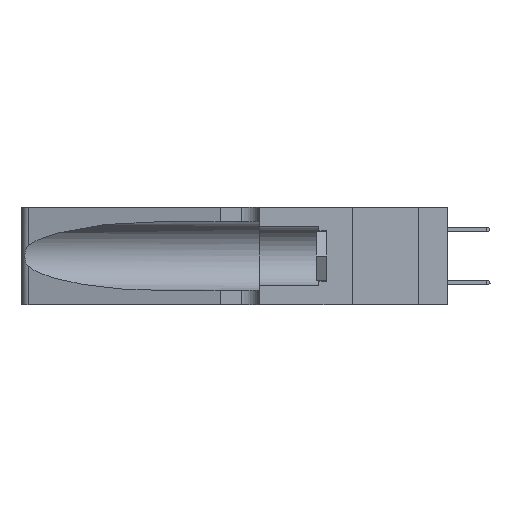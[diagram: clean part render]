
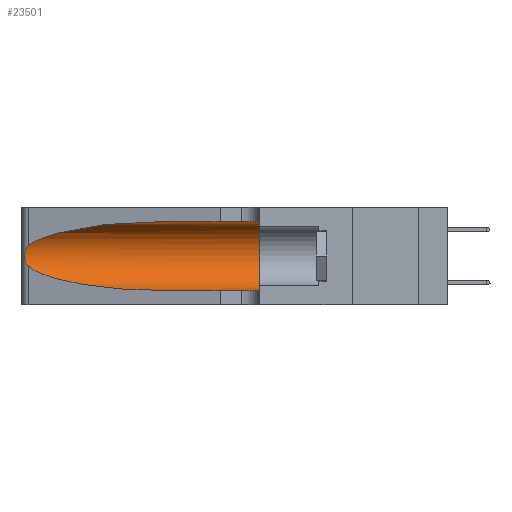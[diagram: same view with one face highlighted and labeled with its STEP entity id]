
A CAD part, left-side view. The second image highlights one B-rep face of the part: STEP entity #23501.
In plain terms, the highlighted cylindrical face has radius 3.308 mm (diameter 6.617 mm), a partial arc.
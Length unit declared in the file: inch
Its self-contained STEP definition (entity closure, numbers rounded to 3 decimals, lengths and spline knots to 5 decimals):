
#346 = CARTESIAN_POINT ( 'NONE',  ( 0.18966, 0.96281, 0.05475 ) ) ;
#382 = CARTESIAN_POINT ( 'NONE',  ( 0.1305, 1.61858, 0.185 ) ) ;
#790 = CARTESIAN_POINT ( 'NONE',  ( 0.1305, 0.72297, 0.31525 ) ) ;
#929 = CARTESIAN_POINT ( 'NONE',  ( 0.25789, 1.23486, 0.15765 ) ) ;
#1046 = CARTESIAN_POINT ( 'NONE',  ( 0.26075, 1.23896, 0.19203 ) ) ;
#2402 = ORIENTED_EDGE ( 'NONE', *, *, #20132, .F. ) ;
#3681 = VECTOR ( 'NONE', #14941, 39.37008 ) ;
#4393 = CARTESIAN_POINT ( 'NONE',  ( 0.25487, 1.22718, 0.22369 ) ) ;
#5688 = CARTESIAN_POINT ( 'NONE',  ( 0.1305, 0.72297, 0.05475 ) ) ;
#6216 = CARTESIAN_POINT ( 'NONE',  ( 0.1305, 1.61858, 0.31525 ) ) ;
#6622 = CARTESIAN_POINT ( 'NONE',  ( 0.25639, 1.23186, 0.15144 ) ) ;
#6860 = CARTESIAN_POINT ( 'NONE',  ( 0.1305, 0.35, 0.185 ) ) ;
#9058 = ORIENTED_EDGE ( 'NONE', *, *, #12781, .T. ) ;
#9461 = CARTESIAN_POINT ( 'NONE',  ( 0.25639, 1.23184, 0.21858 ) ) ;
#9707 = DIRECTION ( 'NONE',  ( 0., 1., 0. ) ) ;
#9995 = ORIENTED_EDGE ( 'NONE', *, *, #31257, .F. ) ;
#11480 = CARTESIAN_POINT ( 'NONE',  ( 0.2373, 1.15595, 0.08982 ) ) ;
#11540 = CARTESIAN_POINT ( 'NONE',  ( 0.1305, 0.72297, 0.31525 ) ) ;
#11659 = CARTESIAN_POINT ( 'NONE',  ( 0.1305, 0.35, 0.05475 ) ) ;
#12025 = CARTESIAN_POINT ( 'NONE',  ( 0.25555, 1.22993, 0.14849 ) ) ;
#12149 = CARTESIAN_POINT ( 'NONE',  ( 0.25854, 1.2359, 0.20912 ) ) ;
#12541 = LINE ( 'NONE', #15565, #25305 ) ;
#12622 = EDGE_CURVE ( 'NONE', #35712, #19726, #35573, .T. ) ;
#12781 = EDGE_CURVE ( 'NONE', #19726, #19125, #35124, .T. ) ;
#12976 = AXIS2_PLACEMENT_3D ( 'NONE', #6860, #9707, #29433 ) ;
#13161 = CARTESIAN_POINT ( 'NONE',  ( 0.1305, 0.35, 0.31525 ) ) ;
#14578 = VERTEX_POINT ( 'NONE', #11659 ) ;
#14941 = DIRECTION ( 'NONE',  ( 0., -1., 0. ) ) ;
#15565 = CARTESIAN_POINT ( 'NONE',  ( 0.1305, 1.61858, 0.05475 ) ) ;
#16082 = EDGE_CURVE ( 'NONE', #19125, #25870, #28475, .T. ) ;
#16121 = EDGE_LOOP ( 'NONE', ( #23765, #9058, #29071, #16289, #9995, #2402 ) ) ;
#16289 = ORIENTED_EDGE ( 'NONE', *, *, #34097, .T. ) ;
#16710 = CARTESIAN_POINT ( 'NONE',  ( 0.1305, 0.72297, 0.05475 ) ) ;
#17772 = DIRECTION ( 'NONE',  ( 0., -1., 0. ) ) ;
#18068 = CARTESIAN_POINT ( 'NONE',  ( 0.25787, 1.23484, 0.2124 ) ) ;
#19125 = VERTEX_POINT ( 'NONE', #36309 ) ;
#19726 = VERTEX_POINT ( 'NONE', #4393 ) ;
#20132 = EDGE_CURVE ( 'NONE', #35712, #32772, #32835, .T. ) ;
#23467 = CARTESIAN_POINT ( 'NONE',  ( 0.25555, 1.22994, 0.2215 ) ) ;
#23501 = ADVANCED_FACE ( 'NONE', ( #26353 ), #27658, .F. ) ;
#23765 = ORIENTED_EDGE ( 'NONE', *, *, #12622, .T. ) ;
#25305 = VECTOR ( 'NONE', #35511, 39.37008 ) ;
#25576 = CARTESIAN_POINT ( 'NONE',  ( 0.2373, 1.15595, 0.28018 ) ) ;
#25870 = VERTEX_POINT ( 'NONE', #16710 ) ;
#26353 = FACE_OUTER_BOUND ( 'NONE', #16121, .T. ) ;
#27658 = CYLINDRICAL_SURFACE ( 'NONE', #36118, 0.13025 ) ;
#28475 =( BOUNDED_CURVE ( )  B_SPLINE_CURVE ( 3, ( #31233, #11480, #346, #5688 ),
 .UNSPECIFIED., .F., .F. ) 
 B_SPLINE_CURVE_WITH_KNOTS ( ( 4, 4 ),
 ( 3.44316, 4.71239 ),
 .UNSPECIFIED. ) 
 CURVE ( )  GEOMETRIC_REPRESENTATION_ITEM ( )  RATIONAL_B_SPLINE_CURVE ( ( 1., 0.87, 0.87, 1. ) ) 
 REPRESENTATION_ITEM ( '' )  );
#28907 = DIRECTION ( 'NONE',  ( 0., 0., -1. ) ) ;
#28951 = CARTESIAN_POINT ( 'NONE',  ( 0.26018, 1.23835, 0.19895 ) ) ;
#29071 = ORIENTED_EDGE ( 'NONE', *, *, #16082, .T. ) ;
#29073 = CARTESIAN_POINT ( 'NONE',  ( 0.25487, 1.22718, 0.22369 ) ) ;
#29151 = CIRCLE ( 'NONE', #12976, 0.13025 ) ;
#29200 = CARTESIAN_POINT ( 'NONE',  ( 0.26075, 1.23896, 0.178 ) ) ;
#29433 = DIRECTION ( 'NONE',  ( 0., 0., 1. ) ) ;
#31180 = CARTESIAN_POINT ( 'NONE',  ( 0.18966, 0.96281, 0.31525 ) ) ;
#31233 = CARTESIAN_POINT ( 'NONE',  ( 0.25487, 1.22718, 0.14631 ) ) ;
#31257 = EDGE_CURVE ( 'NONE', #32772, #14578, #29151, .T. ) ;
#31546 = CARTESIAN_POINT ( 'NONE',  ( 0.25487, 1.22718, 0.22369 ) ) ;
#31926 = CARTESIAN_POINT ( 'NONE',  ( 0.26017, 1.23833, 0.17102 ) ) ;
#32772 = VERTEX_POINT ( 'NONE', #13161 ) ;
#32835 = LINE ( 'NONE', #6216, #3681 ) ;
#34097 = EDGE_CURVE ( 'NONE', #25870, #14578, #12541, .T. ) ;
#34808 = CARTESIAN_POINT ( 'NONE',  ( 0.25856, 1.23593, 0.16098 ) ) ;
#35051 = CARTESIAN_POINT ( 'NONE',  ( 0.25487, 1.22718, 0.14631 ) ) ;
#35124 = B_SPLINE_CURVE_WITH_KNOTS ( 'NONE', 3,
 ( #29073, #23467, #9461, #18068, #12149, #28951, #1046, #29200, #31926, #34808, #929, #6622, #12025, #35051 ),
 .UNSPECIFIED., .F., .F.,
 ( 4, 2, 2, 2, 2, 2, 4 ),
 ( 0., 0.00027, 0.00053, 0.00107, 0.0016, 0.00187, 0.00214 ),
 .UNSPECIFIED. ) ;
#35511 = DIRECTION ( 'NONE',  ( 0., -1., 0. ) ) ;
#35573 =( BOUNDED_CURVE ( )  B_SPLINE_CURVE ( 3, ( #11540, #31180, #25576, #31546 ),
 .UNSPECIFIED., .F., .F. ) 
 B_SPLINE_CURVE_WITH_KNOTS ( ( 4, 4 ),
 ( 1.5708, 2.84003 ),
 .UNSPECIFIED. ) 
 CURVE ( )  GEOMETRIC_REPRESENTATION_ITEM ( )  RATIONAL_B_SPLINE_CURVE ( ( 1., 0.87, 0.87, 1. ) ) 
 REPRESENTATION_ITEM ( '' )  );
#35712 = VERTEX_POINT ( 'NONE', #790 ) ;
#36118 = AXIS2_PLACEMENT_3D ( 'NONE', #382, #17772, #28907 ) ;
#36309 = CARTESIAN_POINT ( 'NONE',  ( 0.25487, 1.22718, 0.14631 ) ) ;
